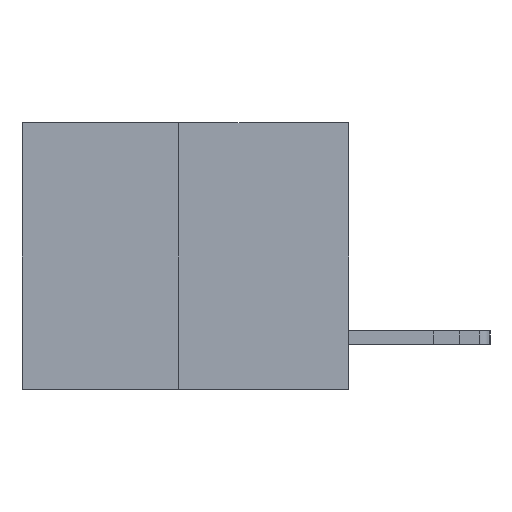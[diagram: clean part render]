
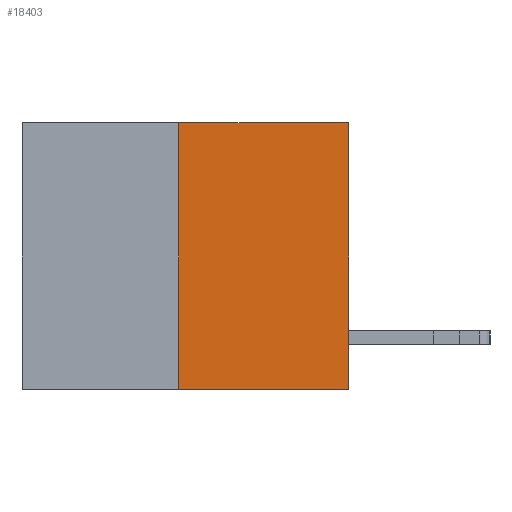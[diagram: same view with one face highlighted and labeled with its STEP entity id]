
A CAD part, left-side view. The second image highlights one B-rep face of the part: STEP entity #18403.
In plain terms, the highlighted planar face has unit normal (-1, 0, 0).
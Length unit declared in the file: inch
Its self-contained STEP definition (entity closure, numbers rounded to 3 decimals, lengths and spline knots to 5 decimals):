
#266 = CARTESIAN_POINT ( 'NONE',  ( 0., 0.6, 0. ) ) ;
#389 = ORIENTED_EDGE ( 'NONE', *, *, #2152, .T. ) ;
#492 = FACE_OUTER_BOUND ( 'NONE', #17073, .T. ) ;
#713 = CARTESIAN_POINT ( 'NONE',  ( 0., 0.6, 0. ) ) ;
#1179 = LINE ( 'NONE', #2878, #11538 ) ;
#1448 = LINE ( 'NONE', #13602, #5590 ) ;
#1623 = VERTEX_POINT ( 'NONE', #5986 ) ;
#1713 = VERTEX_POINT ( 'NONE', #4989 ) ;
#2152 = EDGE_CURVE ( 'NONE', #1713, #9822, #1448, .T. ) ;
#2383 = LINE ( 'NONE', #16115, #4890 ) ;
#2878 = CARTESIAN_POINT ( 'NONE',  ( 0., 0.312, -0.49 ) ) ;
#3140 = EDGE_CURVE ( 'NONE', #1713, #1623, #1179, .T. ) ;
#3228 = DIRECTION ( 'NONE',  ( 0., -1., 0. ) ) ;
#3882 = EDGE_CURVE ( 'NONE', #1623, #12793, #5259, .T. ) ;
#4159 = AXIS2_PLACEMENT_3D ( 'NONE', #713, #13954, #13891 ) ;
#4890 = VECTOR ( 'NONE', #10072, 39.37008 ) ;
#4989 = CARTESIAN_POINT ( 'NONE',  ( 0., 0.312, -0.49 ) ) ;
#5259 = LINE ( 'NONE', #266, #7566 ) ;
#5590 = VECTOR ( 'NONE', #18550, 39.37008 ) ;
#5986 = CARTESIAN_POINT ( 'NONE',  ( 0., 0.312, 0. ) ) ;
#6563 = PLANE ( 'NONE',  #4159 ) ;
#7566 = VECTOR ( 'NONE', #3228, 39.37008 ) ;
#9822 = VERTEX_POINT ( 'NONE', #10938 ) ;
#10038 = DIRECTION ( 'NONE',  ( 0., 0., 1. ) ) ;
#10072 = DIRECTION ( 'NONE',  ( 0., 0., 1. ) ) ;
#10938 = CARTESIAN_POINT ( 'NONE',  ( 0., 0., -0.49 ) ) ;
#11538 = VECTOR ( 'NONE', #10038, 39.37008 ) ;
#12629 = EDGE_CURVE ( 'NONE', #9822, #12793, #2383, .T. ) ;
#12793 = VERTEX_POINT ( 'NONE', #17974 ) ;
#13602 = CARTESIAN_POINT ( 'NONE',  ( 0., 0.6, -0.49 ) ) ;
#13891 = DIRECTION ( 'NONE',  ( 0., 0., -1. ) ) ;
#13954 = DIRECTION ( 'NONE',  ( 1., 0., 0. ) ) ;
#14324 = ORIENTED_EDGE ( 'NONE', *, *, #3140, .F. ) ;
#16115 = CARTESIAN_POINT ( 'NONE',  ( 0., 0., 0. ) ) ;
#16505 = ORIENTED_EDGE ( 'NONE', *, *, #12629, .T. ) ;
#17073 = EDGE_LOOP ( 'NONE', ( #14324, #389, #16505, #17662 ) ) ;
#17662 = ORIENTED_EDGE ( 'NONE', *, *, #3882, .F. ) ;
#17974 = CARTESIAN_POINT ( 'NONE',  ( 0., 0., 0. ) ) ;
#18403 = ADVANCED_FACE ( 'NONE', ( #492 ), #6563, .F. ) ;
#18550 = DIRECTION ( 'NONE',  ( 0., -1., 0. ) ) ;
